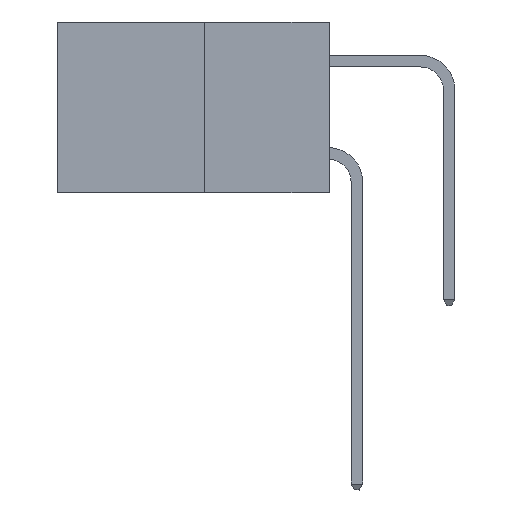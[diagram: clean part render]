
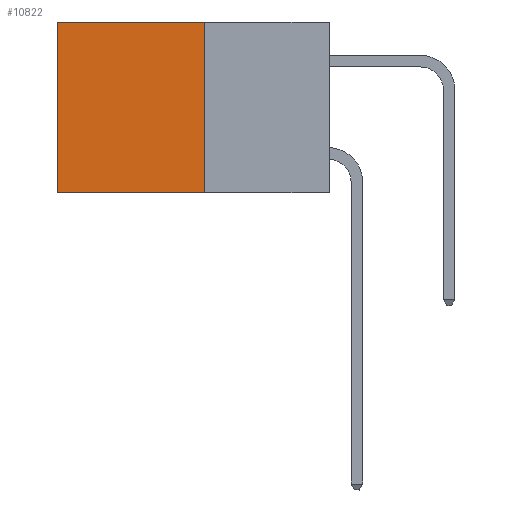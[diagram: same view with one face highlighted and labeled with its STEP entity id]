
A CAD part, left-side view. The second image highlights one B-rep face of the part: STEP entity #10822.
In plain terms, the highlighted planar face has unit normal (-1, 0, 0).
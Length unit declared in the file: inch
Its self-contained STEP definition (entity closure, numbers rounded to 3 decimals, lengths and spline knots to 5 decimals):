
#514 = ORIENTED_EDGE ( 'NONE', *, *, #2819, .F. ) ;
#842 = DIRECTION ( 'NONE',  ( 1., 0., 0. ) ) ;
#916 = ORIENTED_EDGE ( 'NONE', *, *, #7983, .T. ) ;
#2819 = EDGE_CURVE ( 'NONE', #9971, #9456, #10759, .T. ) ;
#3396 = AXIS2_PLACEMENT_3D ( 'NONE', #6149, #842, #8316 ) ;
#4121 = EDGE_LOOP ( 'NONE', ( #8763, #514, #11976, #916 ) ) ;
#4449 = EDGE_CURVE ( 'NONE', #4793, #9971, #8812, .T. ) ;
#4587 = DIRECTION ( 'NONE',  ( 0., 0., -1. ) ) ;
#4605 = CARTESIAN_POINT ( 'NONE',  ( 0.277, 0.59, 0. ) ) ;
#4753 = LINE ( 'NONE', #5599, #10025 ) ;
#4793 = VERTEX_POINT ( 'NONE', #6250 ) ;
#5599 = CARTESIAN_POINT ( 'NONE',  ( 0.277, 0.59, -0.37 ) ) ;
#5662 = VECTOR ( 'NONE', #7770, 39.37008 ) ;
#6149 = CARTESIAN_POINT ( 'NONE',  ( 0.277, 0.27, -0.37 ) ) ;
#6250 = CARTESIAN_POINT ( 'NONE',  ( 0.277, 0.27, 0. ) ) ;
#6520 = CARTESIAN_POINT ( 'NONE',  ( 0.277, 0.27, 0. ) ) ;
#7051 = CARTESIAN_POINT ( 'NONE',  ( 0.277, 0.27, -0.37 ) ) ;
#7770 = DIRECTION ( 'NONE',  ( 0., 0., -1. ) ) ;
#7891 = VECTOR ( 'NONE', #11243, 39.37008 ) ;
#7983 = EDGE_CURVE ( 'NONE', #4793, #9471, #13250, .T. ) ;
#8316 = DIRECTION ( 'NONE',  ( 0., 0., -1. ) ) ;
#8703 = DIRECTION ( 'NONE',  ( 0., 1., 0. ) ) ;
#8763 = ORIENTED_EDGE ( 'NONE', *, *, #10297, .T. ) ;
#8765 = CARTESIAN_POINT ( 'NONE',  ( 0.277, 0.59, -0.37 ) ) ;
#8812 = LINE ( 'NONE', #7051, #5662 ) ;
#9174 = FACE_OUTER_BOUND ( 'NONE', #4121, .T. ) ;
#9456 = VERTEX_POINT ( 'NONE', #8765 ) ;
#9471 = VERTEX_POINT ( 'NONE', #4605 ) ;
#9971 = VERTEX_POINT ( 'NONE', #11548 ) ;
#10025 = VECTOR ( 'NONE', #4587, 39.37008 ) ;
#10082 = VECTOR ( 'NONE', #8703, 39.37008 ) ;
#10297 = EDGE_CURVE ( 'NONE', #9471, #9456, #4753, .T. ) ;
#10759 = LINE ( 'NONE', #11715, #7891 ) ;
#10822 = ADVANCED_FACE ( 'NONE', ( #9174 ), #11528, .F. ) ;
#11243 = DIRECTION ( 'NONE',  ( 0., 1., 0. ) ) ;
#11528 = PLANE ( 'NONE',  #3396 ) ;
#11548 = CARTESIAN_POINT ( 'NONE',  ( 0.277, 0.27, -0.37 ) ) ;
#11715 = CARTESIAN_POINT ( 'NONE',  ( 0.277, 0.27, -0.37 ) ) ;
#11976 = ORIENTED_EDGE ( 'NONE', *, *, #4449, .F. ) ;
#13250 = LINE ( 'NONE', #6520, #10082 ) ;
